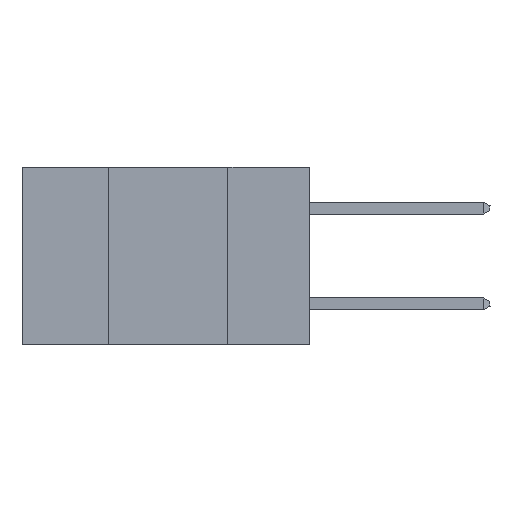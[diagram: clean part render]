
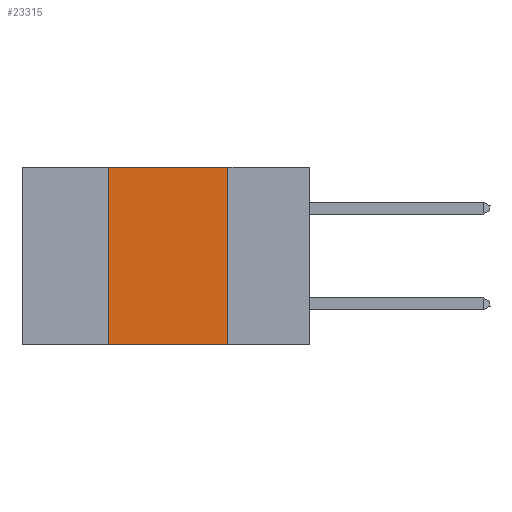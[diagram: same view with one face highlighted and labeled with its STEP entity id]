
A CAD part, left-side view. The second image highlights one B-rep face of the part: STEP entity #23315.
In plain terms, the highlighted planar face has unit normal (-1, 0, 0).
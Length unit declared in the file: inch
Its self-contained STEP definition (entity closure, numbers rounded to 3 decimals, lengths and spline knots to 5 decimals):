
#94 = VERTEX_POINT ( 'NONE', #32281 ) ;
#343 = DIRECTION ( 'NONE',  ( 0., -1., 0. ) ) ;
#652 = ORIENTED_EDGE ( 'NONE', *, *, #23669, .F. ) ;
#749 = EDGE_CURVE ( 'NONE', #41205, #26562, #23456, .T. ) ;
#2093 = VECTOR ( 'NONE', #343, 39.37008 ) ;
#2997 = PLANE ( 'NONE',  #39144 ) ;
#6426 = DIRECTION ( 'NONE',  ( 1., 0., 0. ) ) ;
#6887 = VECTOR ( 'NONE', #12493, 39.37008 ) ;
#7034 = CARTESIAN_POINT ( 'NONE',  ( 0., 0.6, 0. ) ) ;
#8211 = DIRECTION ( 'NONE',  ( 0., 0., -1. ) ) ;
#8339 = LINE ( 'NONE', #24658, #42192 ) ;
#12357 = EDGE_CURVE ( 'NONE', #41205, #94, #39414, .T. ) ;
#12493 = DIRECTION ( 'NONE',  ( 0., 0., 1. ) ) ;
#15930 = ORIENTED_EDGE ( 'NONE', *, *, #12357, .T. ) ;
#18488 = ORIENTED_EDGE ( 'NONE', *, *, #31910, .F. ) ;
#19437 = CARTESIAN_POINT ( 'NONE',  ( 0., 0.42, -0.37 ) ) ;
#20499 = CARTESIAN_POINT ( 'NONE',  ( 0., 0.6, -0.37 ) ) ;
#23315 = ADVANCED_FACE ( 'NONE', ( #38127 ), #2997, .F. ) ;
#23456 = LINE ( 'NONE', #35360, #6887 ) ;
#23669 = EDGE_CURVE ( 'NONE', #25619, #94, #8339, .T. ) ;
#24658 = CARTESIAN_POINT ( 'NONE',  ( 0., 0.17, 0. ) ) ;
#25619 = VERTEX_POINT ( 'NONE', #25870 ) ;
#25870 = CARTESIAN_POINT ( 'NONE',  ( 0., 0.17, 0. ) ) ;
#26562 = VERTEX_POINT ( 'NONE', #36780 ) ;
#28578 = LINE ( 'NONE', #7034, #2093 ) ;
#29525 = DIRECTION ( 'NONE',  ( 0., 0., -1. ) ) ;
#30334 = DIRECTION ( 'NONE',  ( 0., -1., 0. ) ) ;
#31910 = EDGE_CURVE ( 'NONE', #26562, #25619, #28578, .T. ) ;
#32281 = CARTESIAN_POINT ( 'NONE',  ( 0., 0.17, -0.37 ) ) ;
#35360 = CARTESIAN_POINT ( 'NONE',  ( 0., 0.42, 0. ) ) ;
#36780 = CARTESIAN_POINT ( 'NONE',  ( 0., 0.42, 0. ) ) ;
#37884 = ORIENTED_EDGE ( 'NONE', *, *, #749, .F. ) ;
#38127 = FACE_OUTER_BOUND ( 'NONE', #38373, .T. ) ;
#38373 = EDGE_LOOP ( 'NONE', ( #652, #18488, #37884, #15930 ) ) ;
#38393 = VECTOR ( 'NONE', #30334, 39.37008 ) ;
#39144 = AXIS2_PLACEMENT_3D ( 'NONE', #42511, #6426, #29525 ) ;
#39414 = LINE ( 'NONE', #20499, #38393 ) ;
#41205 = VERTEX_POINT ( 'NONE', #19437 ) ;
#42192 = VECTOR ( 'NONE', #8211, 39.37008 ) ;
#42511 = CARTESIAN_POINT ( 'NONE',  ( 0., 0.6, 0. ) ) ;
